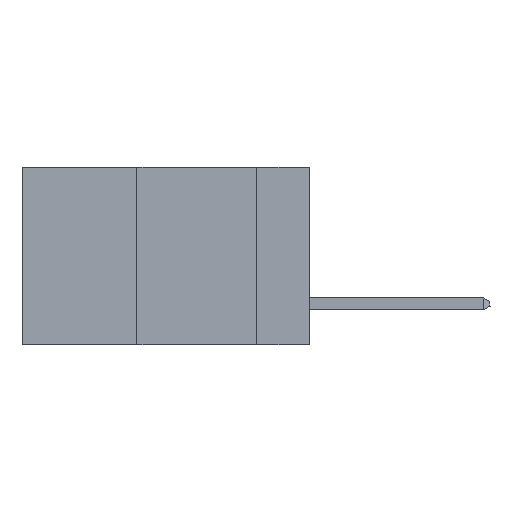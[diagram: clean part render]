
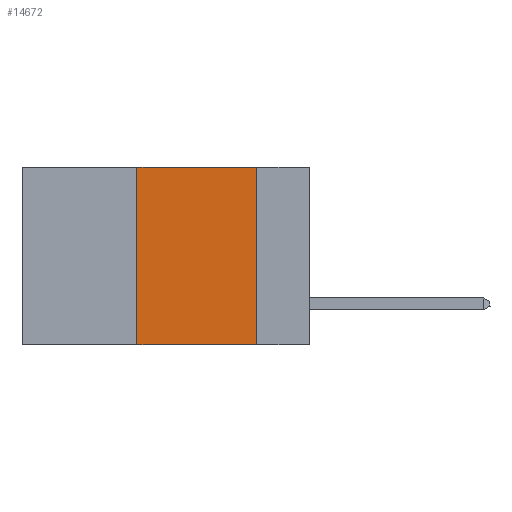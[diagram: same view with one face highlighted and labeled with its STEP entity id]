
A CAD part, left-side view. The second image highlights one B-rep face of the part: STEP entity #14672.
In plain terms, the highlighted planar face has unit normal (-1, 0, 0).
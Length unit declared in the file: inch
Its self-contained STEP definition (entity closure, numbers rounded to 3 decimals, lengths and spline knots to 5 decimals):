
#339 = LINE ( 'NONE', #4132, #1719 ) ;
#806 = VERTEX_POINT ( 'NONE', #11940 ) ;
#1719 = VECTOR ( 'NONE', #14211, 39.37008 ) ;
#1730 = CARTESIAN_POINT ( 'NONE',  ( 0., 0.36, 0. ) ) ;
#2249 = EDGE_CURVE ( 'NONE', #2356, #806, #4360, .T. ) ;
#2356 = VERTEX_POINT ( 'NONE', #1730 ) ;
#2452 = PLANE ( 'NONE',  #4956 ) ;
#3001 = DIRECTION ( 'NONE',  ( 0., -1., 0. ) ) ;
#4132 = CARTESIAN_POINT ( 'NONE',  ( 0., 0.6, -0.37 ) ) ;
#4360 = LINE ( 'NONE', #6715, #16146 ) ;
#4537 = ORIENTED_EDGE ( 'NONE', *, *, #9298, .T. ) ;
#4956 = AXIS2_PLACEMENT_3D ( 'NONE', #12598, #11251, #12528 ) ;
#5070 = LINE ( 'NONE', #15588, #12165 ) ;
#5664 = DIRECTION ( 'NONE',  ( 0., 0., 1. ) ) ;
#6715 = CARTESIAN_POINT ( 'NONE',  ( 0., 0.6, 0. ) ) ;
#6803 = EDGE_CURVE ( 'NONE', #7018, #2356, #8339, .T. ) ;
#7018 = VERTEX_POINT ( 'NONE', #9530 ) ;
#7125 = EDGE_LOOP ( 'NONE', ( #15860, #10384, #13895, #4537 ) ) ;
#8339 = LINE ( 'NONE', #10300, #13047 ) ;
#8436 = VERTEX_POINT ( 'NONE', #8845 ) ;
#8845 = CARTESIAN_POINT ( 'NONE',  ( 0., 0.11, -0.37 ) ) ;
#9298 = EDGE_CURVE ( 'NONE', #7018, #8436, #339, .T. ) ;
#9530 = CARTESIAN_POINT ( 'NONE',  ( 0., 0.36, -0.37 ) ) ;
#9749 = FACE_OUTER_BOUND ( 'NONE', #7125, .T. ) ;
#10300 = CARTESIAN_POINT ( 'NONE',  ( 0., 0.36, 0. ) ) ;
#10384 = ORIENTED_EDGE ( 'NONE', *, *, #2249, .F. ) ;
#11251 = DIRECTION ( 'NONE',  ( 1., 0., 0. ) ) ;
#11940 = CARTESIAN_POINT ( 'NONE',  ( 0., 0.11, 0. ) ) ;
#12165 = VECTOR ( 'NONE', #13110, 39.37008 ) ;
#12528 = DIRECTION ( 'NONE',  ( 0., 0., -1. ) ) ;
#12598 = CARTESIAN_POINT ( 'NONE',  ( 0., 0.6, 0. ) ) ;
#13047 = VECTOR ( 'NONE', #5664, 39.37008 ) ;
#13110 = DIRECTION ( 'NONE',  ( 0., 0., -1. ) ) ;
#13895 = ORIENTED_EDGE ( 'NONE', *, *, #6803, .F. ) ;
#14177 = EDGE_CURVE ( 'NONE', #806, #8436, #5070, .T. ) ;
#14211 = DIRECTION ( 'NONE',  ( 0., -1., 0. ) ) ;
#14672 = ADVANCED_FACE ( 'NONE', ( #9749 ), #2452, .F. ) ;
#15588 = CARTESIAN_POINT ( 'NONE',  ( 0., 0.11, 0. ) ) ;
#15860 = ORIENTED_EDGE ( 'NONE', *, *, #14177, .F. ) ;
#16146 = VECTOR ( 'NONE', #3001, 39.37008 ) ;
